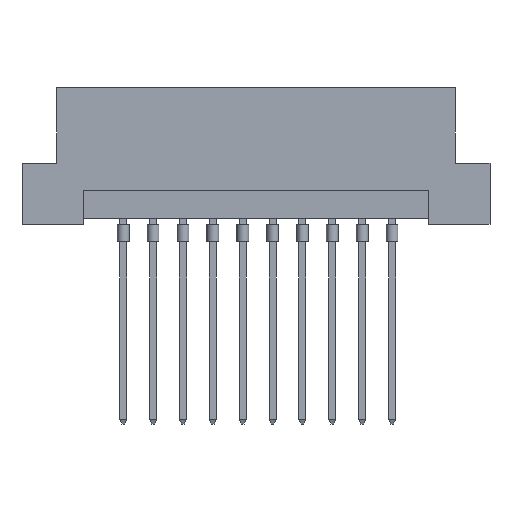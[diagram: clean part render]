
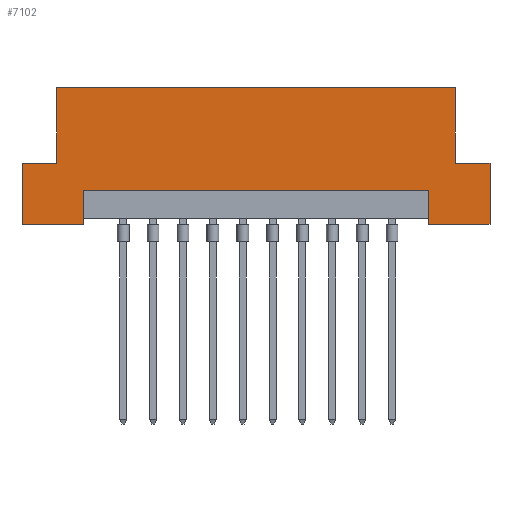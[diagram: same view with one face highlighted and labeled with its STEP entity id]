
A CAD part, front view. The second image highlights one B-rep face of the part: STEP entity #7102.
In plain terms, the highlighted planar face has unit normal (0, -1, 0).
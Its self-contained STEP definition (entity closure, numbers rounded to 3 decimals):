
#68 = DIRECTION ( 'NONE',  ( 0., 0., 1. ) ) ;
#148 = VERTEX_POINT ( 'NONE', #4849 ) ;
#202 = DIRECTION ( 'NONE',  ( 0., 1., 0. ) ) ;
#230 = EDGE_CURVE ( 'NONE', #6411, #5775, #3927, .T. ) ;
#317 = VERTEX_POINT ( 'NONE', #1142 ) ;
#364 = VECTOR ( 'NONE', #4056, 1000. ) ;
#460 = ORIENTED_EDGE ( 'NONE', *, *, #6061, .F. ) ;
#557 = VECTOR ( 'NONE', #837, 1000. ) ;
#613 = EDGE_CURVE ( 'NONE', #6411, #317, #5907, .T. ) ;
#639 = EDGE_CURVE ( 'NONE', #1300, #3959, #719, .T. ) ;
#719 = LINE ( 'NONE', #5984, #6519 ) ;
#837 = DIRECTION ( 'NONE',  ( -1., 0., 0. ) ) ;
#979 = LINE ( 'NONE', #5039, #2816 ) ;
#1015 = LINE ( 'NONE', #2804, #364 ) ;
#1142 = CARTESIAN_POINT ( 'NONE',  ( 14.69, 0., 0. ) ) ;
#1147 = CARTESIAN_POINT ( 'NONE',  ( 16.94, 0., 11.6 ) ) ;
#1155 = VECTOR ( 'NONE', #2836, 1000. ) ;
#1261 = EDGE_CURVE ( 'NONE', #5775, #148, #4927, .T. ) ;
#1300 = VERTEX_POINT ( 'NONE', #5640 ) ;
#1691 = CARTESIAN_POINT ( 'NONE',  ( -16.94, 0., 11.6 ) ) ;
#1704 = LINE ( 'NONE', #6356, #5348 ) ;
#1775 = EDGE_CURVE ( 'NONE', #1300, #4268, #979, .T. ) ;
#1799 = CARTESIAN_POINT ( 'NONE',  ( 19.9, 0., 0. ) ) ;
#1864 = CARTESIAN_POINT ( 'NONE',  ( 19.9, 0., 5.2 ) ) ;
#1919 = DIRECTION ( 'NONE',  ( 0., 0., 1. ) ) ;
#1968 = EDGE_CURVE ( 'NONE', #5417, #7511, #3931, .T. ) ;
#2044 = DIRECTION ( 'NONE',  ( 1., 0., 0. ) ) ;
#2072 = ORIENTED_EDGE ( 'NONE', *, *, #613, .T. ) ;
#2087 = ORIENTED_EDGE ( 'NONE', *, *, #639, .T. ) ;
#2145 = CARTESIAN_POINT ( 'NONE',  ( -19.9, 0., 5.2 ) ) ;
#2260 = LINE ( 'NONE', #6935, #1155 ) ;
#2332 = ORIENTED_EDGE ( 'NONE', *, *, #7090, .F. ) ;
#2542 = CARTESIAN_POINT ( 'NONE',  ( -16.94, 0., 5.2 ) ) ;
#2804 = CARTESIAN_POINT ( 'NONE',  ( -19.9, 0., 11.6 ) ) ;
#2816 = VECTOR ( 'NONE', #2044, 1000. ) ;
#2821 = VERTEX_POINT ( 'NONE', #5611 ) ;
#2836 = DIRECTION ( 'NONE',  ( 0., 0., -1. ) ) ;
#2950 = EDGE_CURVE ( 'NONE', #4268, #6241, #2260, .T. ) ;
#3168 = CARTESIAN_POINT ( 'NONE',  ( 14.69, 0., 2.9 ) ) ;
#3209 = CARTESIAN_POINT ( 'NONE',  ( -16.94, 0., 5.2 ) ) ;
#3278 = DIRECTION ( 'NONE',  ( 0., 0., 1. ) ) ;
#3294 = VECTOR ( 'NONE', #6697, 1000. ) ;
#3327 = DIRECTION ( 'NONE',  ( 1., 0., 0. ) ) ;
#3503 = VERTEX_POINT ( 'NONE', #5738 ) ;
#3597 = EDGE_CURVE ( 'NONE', #148, #3503, #4558, .T. ) ;
#3616 = DIRECTION ( 'NONE',  ( 0., 0., -1. ) ) ;
#3790 = EDGE_CURVE ( 'NONE', #2821, #5417, #6826, .T. ) ;
#3807 = CARTESIAN_POINT ( 'NONE',  ( -14.69, 0., 0.5 ) ) ;
#3821 = ORIENTED_EDGE ( 'NONE', *, *, #230, .F. ) ;
#3927 = LINE ( 'NONE', #3168, #557 ) ;
#3931 = LINE ( 'NONE', #3209, #6834 ) ;
#3959 = VERTEX_POINT ( 'NONE', #1147 ) ;
#3994 = ORIENTED_EDGE ( 'NONE', *, *, #2950, .F. ) ;
#4056 = DIRECTION ( 'NONE',  ( 1., 0., 0. ) ) ;
#4098 = ORIENTED_EDGE ( 'NONE', *, *, #3597, .F. ) ;
#4125 = CARTESIAN_POINT ( 'NONE',  ( -19.9, 0., 0. ) ) ;
#4167 = ORIENTED_EDGE ( 'NONE', *, *, #6056, .F. ) ;
#4243 = CARTESIAN_POINT ( 'NONE',  ( -19.9, 0., 11.6 ) ) ;
#4268 = VERTEX_POINT ( 'NONE', #1864 ) ;
#4478 = DIRECTION ( 'NONE',  ( -1., 0., 0. ) ) ;
#4558 = LINE ( 'NONE', #4125, #5036 ) ;
#4668 = DIRECTION ( 'NONE',  ( -1., 0., 0. ) ) ;
#4759 = PLANE ( 'NONE',  #4862 ) ;
#4849 = CARTESIAN_POINT ( 'NONE',  ( -14.69, 0., 0. ) ) ;
#4862 = AXIS2_PLACEMENT_3D ( 'NONE', #4243, #202, #1919 ) ;
#4927 = LINE ( 'NONE', #3807, #3294 ) ;
#4980 = CARTESIAN_POINT ( 'NONE',  ( 14.69, 0., 2.9 ) ) ;
#5036 = VECTOR ( 'NONE', #4668, 1000. ) ;
#5039 = CARTESIAN_POINT ( 'NONE',  ( 19.9, 0., 5.2 ) ) ;
#5308 = CARTESIAN_POINT ( 'NONE',  ( 14.69, 0., 0.5 ) ) ;
#5348 = VECTOR ( 'NONE', #6961, 1000. ) ;
#5367 = FACE_OUTER_BOUND ( 'NONE', #6640, .T. ) ;
#5417 = VERTEX_POINT ( 'NONE', #2542 ) ;
#5611 = CARTESIAN_POINT ( 'NONE',  ( -19.9, 0., 5.2 ) ) ;
#5640 = CARTESIAN_POINT ( 'NONE',  ( 16.94, 0., 5.2 ) ) ;
#5721 = VECTOR ( 'NONE', #4478, 1000. ) ;
#5738 = CARTESIAN_POINT ( 'NONE',  ( -19.9, 0., 0. ) ) ;
#5775 = VERTEX_POINT ( 'NONE', #5863 ) ;
#5863 = CARTESIAN_POINT ( 'NONE',  ( -14.69, 0., 2.9 ) ) ;
#5907 = LINE ( 'NONE', #5308, #6036 ) ;
#5984 = CARTESIAN_POINT ( 'NONE',  ( 16.94, 0., 5.2 ) ) ;
#5985 = ORIENTED_EDGE ( 'NONE', *, *, #1261, .F. ) ;
#6036 = VECTOR ( 'NONE', #3616, 1000. ) ;
#6056 = EDGE_CURVE ( 'NONE', #7511, #3959, #1015, .T. ) ;
#6061 = EDGE_CURVE ( 'NONE', #6241, #317, #7388, .T. ) ;
#6241 = VERTEX_POINT ( 'NONE', #1799 ) ;
#6303 = ORIENTED_EDGE ( 'NONE', *, *, #3790, .F. ) ;
#6348 = CARTESIAN_POINT ( 'NONE',  ( -19.9, 0., 0. ) ) ;
#6356 = CARTESIAN_POINT ( 'NONE',  ( -19.9, 0., 0. ) ) ;
#6411 = VERTEX_POINT ( 'NONE', #4980 ) ;
#6519 = VECTOR ( 'NONE', #68, 1000. ) ;
#6618 = ORIENTED_EDGE ( 'NONE', *, *, #1968, .F. ) ;
#6640 = EDGE_LOOP ( 'NONE', ( #3821, #2072, #460, #3994, #7161, #2087, #4167, #6618, #6303, #2332, #4098, #5985 ) ) ;
#6697 = DIRECTION ( 'NONE',  ( 0., 0., -1. ) ) ;
#6826 = LINE ( 'NONE', #2145, #7349 ) ;
#6834 = VECTOR ( 'NONE', #3278, 1000. ) ;
#6935 = CARTESIAN_POINT ( 'NONE',  ( 19.9, 0., 0. ) ) ;
#6961 = DIRECTION ( 'NONE',  ( 0., 0., 1. ) ) ;
#7090 = EDGE_CURVE ( 'NONE', #3503, #2821, #1704, .T. ) ;
#7102 = ADVANCED_FACE ( 'NONE', ( #5367 ), #4759, .F. ) ;
#7161 = ORIENTED_EDGE ( 'NONE', *, *, #1775, .F. ) ;
#7349 = VECTOR ( 'NONE', #3327, 1000. ) ;
#7388 = LINE ( 'NONE', #6348, #5721 ) ;
#7511 = VERTEX_POINT ( 'NONE', #1691 ) ;
